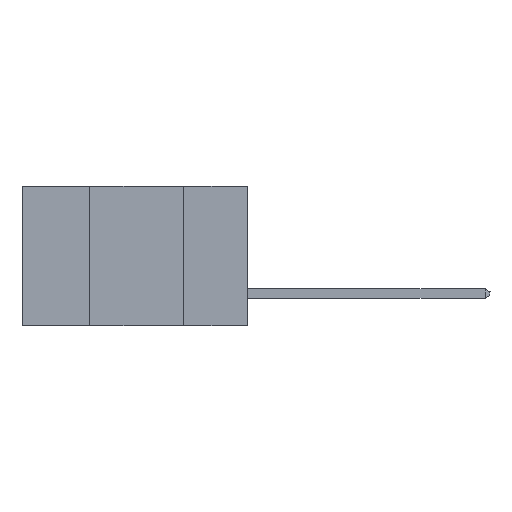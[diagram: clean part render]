
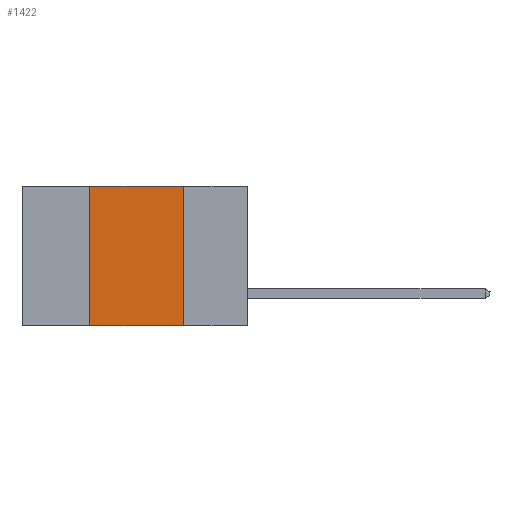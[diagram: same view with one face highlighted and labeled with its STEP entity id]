
A CAD part, left-side view. The second image highlights one B-rep face of the part: STEP entity #1422.
In plain terms, the highlighted planar face has unit normal (-1, 0, 0).
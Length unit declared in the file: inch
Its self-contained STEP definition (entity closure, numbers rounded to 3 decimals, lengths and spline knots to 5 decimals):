
#34 = EDGE_CURVE ( 'NONE', #10308, #12917, #120, .T. ) ;
#120 = LINE ( 'NONE', #6909, #13426 ) ;
#1005 = VERTEX_POINT ( 'NONE', #5669 ) ;
#1422 = ADVANCED_FACE ( 'NONE', ( #11706 ), #7077, .F. ) ;
#1467 = LINE ( 'NONE', #13893, #9639 ) ;
#2166 = DIRECTION ( 'NONE',  ( 0., 0., -1. ) ) ;
#2675 = DIRECTION ( 'NONE',  ( 1., 0., 0. ) ) ;
#3393 = LINE ( 'NONE', #7820, #12729 ) ;
#3475 = CARTESIAN_POINT ( 'NONE',  ( 0., 0.6, 0. ) ) ;
#3678 = ORIENTED_EDGE ( 'NONE', *, *, #6782, .F. ) ;
#3905 = CARTESIAN_POINT ( 'NONE',  ( 0., 0.42, 0. ) ) ;
#4645 = AXIS2_PLACEMENT_3D ( 'NONE', #3475, #2675, #8036 ) ;
#4844 = EDGE_LOOP ( 'NONE', ( #10246, #3678, #12170, #10520 ) ) ;
#5077 = LINE ( 'NONE', #9627, #13229 ) ;
#5258 = EDGE_CURVE ( 'NONE', #1005, #7650, #3393, .T. ) ;
#5669 = CARTESIAN_POINT ( 'NONE',  ( 0., 0.17, 0. ) ) ;
#5897 = EDGE_CURVE ( 'NONE', #10308, #7650, #5077, .T. ) ;
#6002 = DIRECTION ( 'NONE',  ( 0., -1., 0. ) ) ;
#6782 = EDGE_CURVE ( 'NONE', #12917, #1005, #1467, .T. ) ;
#6909 = CARTESIAN_POINT ( 'NONE',  ( 0., 0.42, -0.37 ) ) ;
#7077 = PLANE ( 'NONE',  #4645 ) ;
#7650 = VERTEX_POINT ( 'NONE', #8066 ) ;
#7820 = CARTESIAN_POINT ( 'NONE',  ( 0., 0.17, -0.37 ) ) ;
#8036 = DIRECTION ( 'NONE',  ( 0., 0., -1. ) ) ;
#8066 = CARTESIAN_POINT ( 'NONE',  ( 0., 0.17, -0.37 ) ) ;
#9627 = CARTESIAN_POINT ( 'NONE',  ( 0., 0.6, -0.37 ) ) ;
#9639 = VECTOR ( 'NONE', #6002, 39.37008 ) ;
#10246 = ORIENTED_EDGE ( 'NONE', *, *, #5258, .F. ) ;
#10308 = VERTEX_POINT ( 'NONE', #10457 ) ;
#10457 = CARTESIAN_POINT ( 'NONE',  ( 0., 0.42, -0.37 ) ) ;
#10520 = ORIENTED_EDGE ( 'NONE', *, *, #5897, .T. ) ;
#11706 = FACE_OUTER_BOUND ( 'NONE', #4844, .T. ) ;
#12170 = ORIENTED_EDGE ( 'NONE', *, *, #34, .F. ) ;
#12729 = VECTOR ( 'NONE', #2166, 39.37008 ) ;
#12917 = VERTEX_POINT ( 'NONE', #3905 ) ;
#13229 = VECTOR ( 'NONE', #14214, 39.37008 ) ;
#13426 = VECTOR ( 'NONE', #13737, 39.37008 ) ;
#13737 = DIRECTION ( 'NONE',  ( 0., 0., 1. ) ) ;
#13893 = CARTESIAN_POINT ( 'NONE',  ( 0., 0.6, 0. ) ) ;
#14214 = DIRECTION ( 'NONE',  ( 0., -1., 0. ) ) ;
